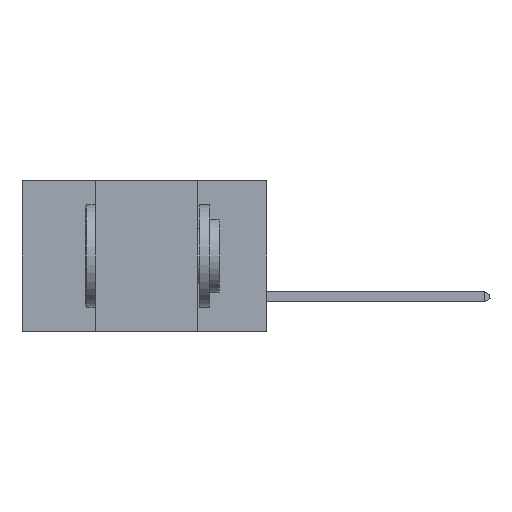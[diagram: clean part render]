
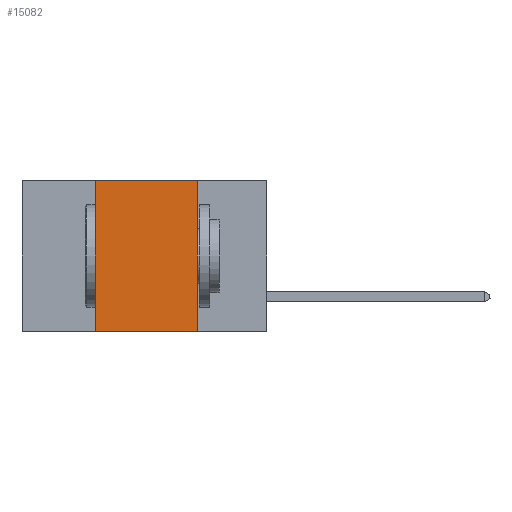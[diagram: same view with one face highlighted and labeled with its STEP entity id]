
A CAD part, left-side view. The second image highlights one B-rep face of the part: STEP entity #15082.
In plain terms, the highlighted planar face has unit normal (-1, 0, 0).
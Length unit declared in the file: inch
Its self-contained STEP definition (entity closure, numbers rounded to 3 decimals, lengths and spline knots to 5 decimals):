
#2097 = ORIENTED_EDGE ( 'NONE', *, *, #3570, .F. ) ;
#3570 = EDGE_CURVE ( 'NONE', #22823, #22955, #11910, .T. ) ;
#3585 = VECTOR ( 'NONE', #3745, 39.37008 ) ;
#3745 = DIRECTION ( 'NONE',  ( 0., -1., 0. ) ) ;
#4818 = CARTESIAN_POINT ( 'NONE',  ( 0., 0.42, -0.37 ) ) ;
#6373 = EDGE_CURVE ( 'NONE', #22955, #13659, #35151, .T. ) ;
#7569 = DIRECTION ( 'NONE',  ( 0., 0., 1. ) ) ;
#8008 = EDGE_CURVE ( 'NONE', #22823, #10712, #10641, .T. ) ;
#8180 = CARTESIAN_POINT ( 'NONE',  ( 0., 0.6, -0.37 ) ) ;
#8209 = CARTESIAN_POINT ( 'NONE',  ( 0., 0.42, 0. ) ) ;
#8899 = PLANE ( 'NONE',  #34516 ) ;
#9879 = CARTESIAN_POINT ( 'NONE',  ( 0., 0.6, 0. ) ) ;
#10467 = CARTESIAN_POINT ( 'NONE',  ( 0., 0.42, 0. ) ) ;
#10572 = CARTESIAN_POINT ( 'NONE',  ( 0., 0.17, 0. ) ) ;
#10641 = LINE ( 'NONE', #8180, #27283 ) ;
#10712 = VERTEX_POINT ( 'NONE', #27313 ) ;
#10950 = DIRECTION ( 'NONE',  ( 0., -1., 0. ) ) ;
#11670 = DIRECTION ( 'NONE',  ( 0., 0., -1. ) ) ;
#11910 = LINE ( 'NONE', #10467, #36264 ) ;
#12681 = LINE ( 'NONE', #18833, #14445 ) ;
#13659 = VERTEX_POINT ( 'NONE', #10572 ) ;
#14022 = EDGE_LOOP ( 'NONE', ( #14813, #21212, #2097, #25194 ) ) ;
#14445 = VECTOR ( 'NONE', #24345, 39.37008 ) ;
#14813 = ORIENTED_EDGE ( 'NONE', *, *, #27357, .F. ) ;
#15082 = ADVANCED_FACE ( 'NONE', ( #32272 ), #8899, .F. ) ;
#18833 = CARTESIAN_POINT ( 'NONE',  ( 0., 0.17, 0. ) ) ;
#21212 = ORIENTED_EDGE ( 'NONE', *, *, #6373, .F. ) ;
#22823 = VERTEX_POINT ( 'NONE', #4818 ) ;
#22955 = VERTEX_POINT ( 'NONE', #8209 ) ;
#24345 = DIRECTION ( 'NONE',  ( 0., 0., -1. ) ) ;
#25194 = ORIENTED_EDGE ( 'NONE', *, *, #8008, .T. ) ;
#27283 = VECTOR ( 'NONE', #10950, 39.37008 ) ;
#27313 = CARTESIAN_POINT ( 'NONE',  ( 0., 0.17, -0.37 ) ) ;
#27357 = EDGE_CURVE ( 'NONE', #13659, #10712, #12681, .T. ) ;
#29167 = CARTESIAN_POINT ( 'NONE',  ( 0., 0.6, 0. ) ) ;
#31704 = DIRECTION ( 'NONE',  ( 1., 0., 0. ) ) ;
#32272 = FACE_OUTER_BOUND ( 'NONE', #14022, .T. ) ;
#34516 = AXIS2_PLACEMENT_3D ( 'NONE', #29167, #31704, #11670 ) ;
#35151 = LINE ( 'NONE', #9879, #3585 ) ;
#36264 = VECTOR ( 'NONE', #7569, 39.37008 ) ;
